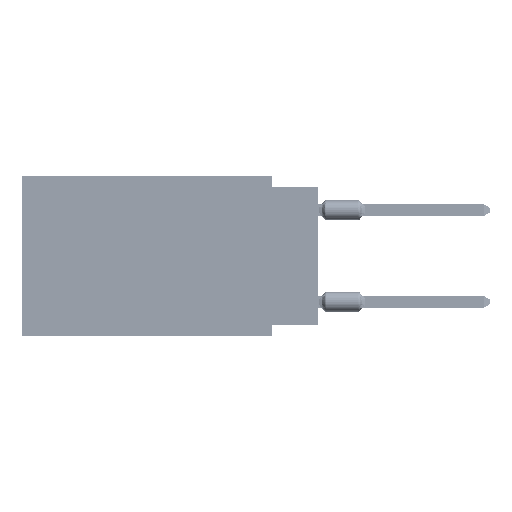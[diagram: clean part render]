
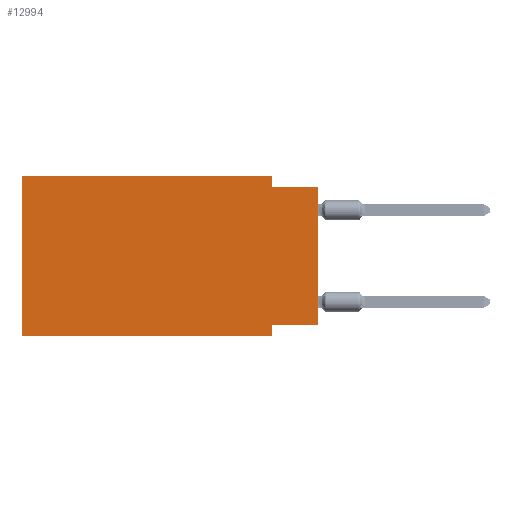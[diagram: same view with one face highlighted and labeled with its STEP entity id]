
A CAD part, left-side view. The second image highlights one B-rep face of the part: STEP entity #12994.
In plain terms, the highlighted planar face has unit normal (-1, 0, 0).
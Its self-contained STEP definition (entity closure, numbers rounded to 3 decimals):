
#695 = DIRECTION ( 'NONE',  ( 0., 0., 1. ) ) ;
#1096 = CARTESIAN_POINT ( 'NONE',  ( 0., 16.383, -8.89 ) ) ;
#1201 = EDGE_CURVE ( 'NONE', #51687, #58347, #1388, .T. ) ;
#1388 = LINE ( 'NONE', #32526, #67283 ) ;
#2117 = PLANE ( 'NONE',  #44239 ) ;
#4349 = ORIENTED_EDGE ( 'NONE', *, *, #63353, .F. ) ;
#4558 = DIRECTION ( 'NONE',  ( 0., 1., 0. ) ) ;
#6047 = VECTOR ( 'NONE', #63373, 1000. ) ;
#7249 = CARTESIAN_POINT ( 'NONE',  ( 0., 0., -8.255 ) ) ;
#8392 = FACE_OUTER_BOUND ( 'NONE', #55289, .T. ) ;
#8563 = LINE ( 'NONE', #30591, #41986 ) ;
#9502 = CARTESIAN_POINT ( 'NONE',  ( 0., 0., -0.635 ) ) ;
#10450 = CARTESIAN_POINT ( 'NONE',  ( 0., 2.54, -8.89 ) ) ;
#10788 = EDGE_CURVE ( 'NONE', #51687, #34443, #17049, .T. ) ;
#12994 = ADVANCED_FACE ( 'NONE', ( #8392 ), #2117, .F. ) ;
#13643 = CARTESIAN_POINT ( 'NONE',  ( 0., 16.383, 0. ) ) ;
#14768 = ORIENTED_EDGE ( 'NONE', *, *, #62972, .F. ) ;
#15043 = VERTEX_POINT ( 'NONE', #44591 ) ;
#17049 = LINE ( 'NONE', #42610, #68655 ) ;
#19479 = ORIENTED_EDGE ( 'NONE', *, *, #67016, .F. ) ;
#19642 = VERTEX_POINT ( 'NONE', #45708 ) ;
#20543 = VECTOR ( 'NONE', #68376, 1000. ) ;
#21039 = ORIENTED_EDGE ( 'NONE', *, *, #22380, .F. ) ;
#22380 = EDGE_CURVE ( 'NONE', #68978, #41573, #48515, .T. ) ;
#23935 = ORIENTED_EDGE ( 'NONE', *, *, #35748, .T. ) ;
#25551 = CARTESIAN_POINT ( 'NONE',  ( 0., 0., -8.255 ) ) ;
#30328 = VECTOR ( 'NONE', #47302, 1000. ) ;
#30591 = CARTESIAN_POINT ( 'NONE',  ( 0., 16.383, 0. ) ) ;
#32526 = CARTESIAN_POINT ( 'NONE',  ( 0., 16.383, 0. ) ) ;
#34391 = CARTESIAN_POINT ( 'NONE',  ( 0., 2.54, -8.89 ) ) ;
#34443 = VERTEX_POINT ( 'NONE', #34391 ) ;
#35748 = EDGE_CURVE ( 'NONE', #68978, #19642, #42408, .T. ) ;
#36804 = ORIENTED_EDGE ( 'NONE', *, *, #10788, .T. ) ;
#37722 = LINE ( 'NONE', #10450, #46378 ) ;
#38138 = CARTESIAN_POINT ( 'NONE',  ( 0., 2.54, 0. ) ) ;
#38387 = DIRECTION ( 'NONE',  ( 0., -1., 0. ) ) ;
#40055 = DIRECTION ( 'NONE',  ( 0., -1., 0. ) ) ;
#40224 = DIRECTION ( 'NONE',  ( 0., 0., -1. ) ) ;
#41573 = VERTEX_POINT ( 'NONE', #54390 ) ;
#41986 = VECTOR ( 'NONE', #40055, 1000. ) ;
#42408 = LINE ( 'NONE', #45674, #30328 ) ;
#42610 = CARTESIAN_POINT ( 'NONE',  ( 0., 16.383, -8.89 ) ) ;
#42981 = EDGE_CURVE ( 'NONE', #58347, #49179, #8563, .T. ) ;
#44239 = AXIS2_PLACEMENT_3D ( 'NONE', #45468, #66825, #40224 ) ;
#44591 = CARTESIAN_POINT ( 'NONE',  ( 0., 2.54, -0.635 ) ) ;
#45468 = CARTESIAN_POINT ( 'NONE',  ( 0., 16.383, 0. ) ) ;
#45674 = CARTESIAN_POINT ( 'NONE',  ( 0., 0., 0. ) ) ;
#45708 = CARTESIAN_POINT ( 'NONE',  ( 0., 0., -0.635 ) ) ;
#45738 = ORIENTED_EDGE ( 'NONE', *, *, #1201, .F. ) ;
#46378 = VECTOR ( 'NONE', #47171, 1000. ) ;
#47012 = CARTESIAN_POINT ( 'NONE',  ( 0., 2.54, 0. ) ) ;
#47171 = DIRECTION ( 'NONE',  ( 0., 0., -1. ) ) ;
#47302 = DIRECTION ( 'NONE',  ( 0., 0., 1. ) ) ;
#48515 = LINE ( 'NONE', #25551, #58334 ) ;
#49179 = VERTEX_POINT ( 'NONE', #38138 ) ;
#51687 = VERTEX_POINT ( 'NONE', #1096 ) ;
#52179 = LINE ( 'NONE', #9502, #6047 ) ;
#54390 = CARTESIAN_POINT ( 'NONE',  ( 0., 2.54, -8.255 ) ) ;
#55289 = EDGE_LOOP ( 'NONE', ( #23935, #4349, #14768, #55992, #45738, #36804, #19479, #21039 ) ) ;
#55992 = ORIENTED_EDGE ( 'NONE', *, *, #42981, .F. ) ;
#58334 = VECTOR ( 'NONE', #4558, 1000. ) ;
#58347 = VERTEX_POINT ( 'NONE', #13643 ) ;
#62972 = EDGE_CURVE ( 'NONE', #49179, #15043, #63808, .T. ) ;
#63353 = EDGE_CURVE ( 'NONE', #15043, #19642, #52179, .T. ) ;
#63373 = DIRECTION ( 'NONE',  ( 0., -1., 0. ) ) ;
#63808 = LINE ( 'NONE', #47012, #20543 ) ;
#66825 = DIRECTION ( 'NONE',  ( 1., 0., 0. ) ) ;
#67016 = EDGE_CURVE ( 'NONE', #41573, #34443, #37722, .T. ) ;
#67283 = VECTOR ( 'NONE', #695, 1000. ) ;
#68376 = DIRECTION ( 'NONE',  ( 0., 0., -1. ) ) ;
#68655 = VECTOR ( 'NONE', #38387, 1000. ) ;
#68978 = VERTEX_POINT ( 'NONE', #7249 ) ;
